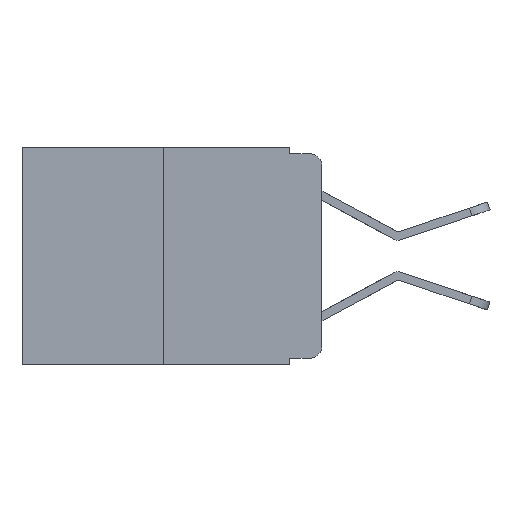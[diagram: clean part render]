
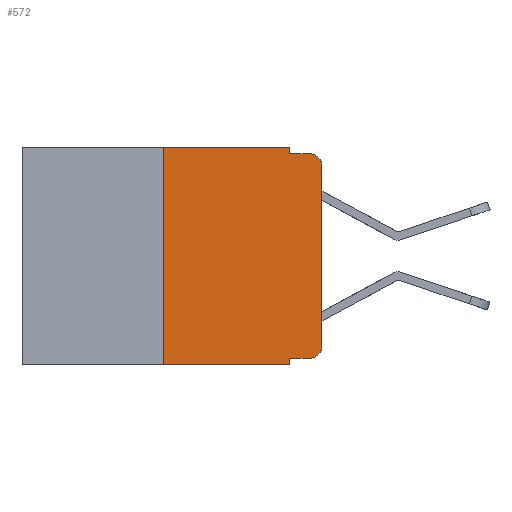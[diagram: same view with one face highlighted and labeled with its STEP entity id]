
A CAD part, left-side view. The second image highlights one B-rep face of the part: STEP entity #572.
In plain terms, the highlighted planar face has unit normal (-1, 0, 0).
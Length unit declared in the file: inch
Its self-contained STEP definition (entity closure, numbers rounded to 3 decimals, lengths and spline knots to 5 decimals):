
#12 = LINE ( 'NONE', #513, #7701 ) ;
#178 = LINE ( 'NONE', #8583, #9653 ) ;
#316 = VERTEX_POINT ( 'NONE', #3952 ) ;
#413 = DIRECTION ( 'NONE',  ( 0., 0., -1. ) ) ;
#513 = CARTESIAN_POINT ( 'NONE',  ( 0., 0.473, -0.343 ) ) ;
#572 = ADVANCED_FACE ( 'NONE', ( #7696 ), #1728, .F. ) ;
#573 = CIRCLE ( 'NONE', #2050, 0.02 ) ;
#633 = ORIENTED_EDGE ( 'NONE', *, *, #4874, .T. ) ;
#648 = ORIENTED_EDGE ( 'NONE', *, *, #5031, .T. ) ;
#751 = VECTOR ( 'NONE', #11041, 39.37008 ) ;
#838 = LINE ( 'NONE', #3670, #3539 ) ;
#1110 = ORIENTED_EDGE ( 'NONE', *, *, #4892, .F. ) ;
#1284 = DIRECTION ( 'NONE',  ( 0., 0., -1. ) ) ;
#1434 = VECTOR ( 'NONE', #4374, 39.37008 ) ;
#1572 = DIRECTION ( 'NONE',  ( 0., -1., 0. ) ) ;
#1720 = CARTESIAN_POINT ( 'NONE',  ( 0., 0.051, 0. ) ) ;
#1728 = PLANE ( 'NONE',  #8110 ) ;
#1743 = ORIENTED_EDGE ( 'NONE', *, *, #4982, .F. ) ;
#1760 = DIRECTION ( 'NONE',  ( 0., -1., 0. ) ) ;
#1807 = ORIENTED_EDGE ( 'NONE', *, *, #5016, .F. ) ;
#2050 = AXIS2_PLACEMENT_3D ( 'NONE', #3298, #6949, #1284 ) ;
#2404 = VERTEX_POINT ( 'NONE', #2656 ) ;
#2656 = CARTESIAN_POINT ( 'NONE',  ( 0., 0.25, -0.343 ) ) ;
#3298 = CARTESIAN_POINT ( 'NONE',  ( 0., 0.02, -0.03 ) ) ;
#3376 = ORIENTED_EDGE ( 'NONE', *, *, #3621, .F. ) ;
#3381 = EDGE_LOOP ( 'NONE', ( #5494, #633, #5001, #1110, #3376, #1743, #6502, #1807, #8353, #648 ) ) ;
#3450 = CARTESIAN_POINT ( 'NONE',  ( 0., 0.25, 0. ) ) ;
#3536 = CARTESIAN_POINT ( 'NONE',  ( 0., 0.051, 0. ) ) ;
#3539 = VECTOR ( 'NONE', #1760, 39.37008 ) ;
#3621 = EDGE_CURVE ( 'NONE', #316, #7828, #838, .T. ) ;
#3670 = CARTESIAN_POINT ( 'NONE',  ( 0., 0.473, 0. ) ) ;
#3745 = DIRECTION ( 'NONE',  ( -1., 0., 0. ) ) ;
#3952 = CARTESIAN_POINT ( 'NONE',  ( 0., 0.25, 0. ) ) ;
#4086 = CARTESIAN_POINT ( 'NONE',  ( 0., 0.051, -0.343 ) ) ;
#4167 = EDGE_CURVE ( 'NONE', #2404, #6299, #12, .T. ) ;
#4369 = LINE ( 'NONE', #3450, #1434 ) ;
#4374 = DIRECTION ( 'NONE',  ( 0., 0., 1. ) ) ;
#4548 = EDGE_CURVE ( 'NONE', #6968, #5547, #11079, .T. ) ;
#4633 = DIRECTION ( 'NONE',  ( 0., 0., -1. ) ) ;
#4672 = DIRECTION ( 'NONE',  ( 1., 0., 0. ) ) ;
#4874 = EDGE_CURVE ( 'NONE', #5547, #6162, #573, .T. ) ;
#4877 = EDGE_CURVE ( 'NONE', #5448, #6162, #178, .T. ) ;
#4892 = EDGE_CURVE ( 'NONE', #7828, #5448, #7560, .T. ) ;
#4982 = EDGE_CURVE ( 'NONE', #2404, #316, #4369, .T. ) ;
#5001 = ORIENTED_EDGE ( 'NONE', *, *, #4877, .F. ) ;
#5016 = EDGE_CURVE ( 'NONE', #8729, #6299, #6192, .T. ) ;
#5019 = EDGE_CURVE ( 'NONE', #8729, #9966, #8169, .T. ) ;
#5031 = EDGE_CURVE ( 'NONE', #9966, #6968, #10485, .T. ) ;
#5239 = AXIS2_PLACEMENT_3D ( 'NONE', #8963, #3745, #7965 ) ;
#5276 = CARTESIAN_POINT ( 'NONE',  ( 0., 0.02, -0.01 ) ) ;
#5448 = VERTEX_POINT ( 'NONE', #5880 ) ;
#5494 = ORIENTED_EDGE ( 'NONE', *, *, #4548, .T. ) ;
#5547 = VERTEX_POINT ( 'NONE', #10273 ) ;
#5880 = CARTESIAN_POINT ( 'NONE',  ( 0., 0.051, -0.01 ) ) ;
#5909 = VECTOR ( 'NONE', #9296, 39.37008 ) ;
#6162 = VERTEX_POINT ( 'NONE', #5276 ) ;
#6192 = LINE ( 'NONE', #3536, #5909 ) ;
#6299 = VERTEX_POINT ( 'NONE', #4086 ) ;
#6502 = ORIENTED_EDGE ( 'NONE', *, *, #4167, .T. ) ;
#6785 = DIRECTION ( 'NONE',  ( 0., -1., 0. ) ) ;
#6922 = VECTOR ( 'NONE', #10106, 39.37008 ) ;
#6949 = DIRECTION ( 'NONE',  ( -1., 0., 0. ) ) ;
#6968 = VERTEX_POINT ( 'NONE', #7885 ) ;
#7242 = CARTESIAN_POINT ( 'NONE',  ( 0., 0.051, -0.333 ) ) ;
#7469 = CARTESIAN_POINT ( 'NONE',  ( 0., 0., 0. ) ) ;
#7560 = LINE ( 'NONE', #1720, #9422 ) ;
#7696 = FACE_OUTER_BOUND ( 'NONE', #3381, .T. ) ;
#7701 = VECTOR ( 'NONE', #1572, 39.37008 ) ;
#7828 = VERTEX_POINT ( 'NONE', #10787 ) ;
#7885 = CARTESIAN_POINT ( 'NONE',  ( 0., 0., -0.313 ) ) ;
#7965 = DIRECTION ( 'NONE',  ( 0., 0., -1. ) ) ;
#8110 = AXIS2_PLACEMENT_3D ( 'NONE', #11077, #4672, #4633 ) ;
#8169 = LINE ( 'NONE', #9331, #751 ) ;
#8353 = ORIENTED_EDGE ( 'NONE', *, *, #5019, .T. ) ;
#8583 = CARTESIAN_POINT ( 'NONE',  ( 0., 0.051, -0.01 ) ) ;
#8729 = VERTEX_POINT ( 'NONE', #7242 ) ;
#8963 = CARTESIAN_POINT ( 'NONE',  ( 0., 0.02, -0.313 ) ) ;
#9296 = DIRECTION ( 'NONE',  ( 0., 0., -1. ) ) ;
#9331 = CARTESIAN_POINT ( 'NONE',  ( 0., 0.051, -0.333 ) ) ;
#9422 = VECTOR ( 'NONE', #413, 39.37008 ) ;
#9653 = VECTOR ( 'NONE', #6785, 39.37008 ) ;
#9966 = VERTEX_POINT ( 'NONE', #11499 ) ;
#10106 = DIRECTION ( 'NONE',  ( 0., 0., 1. ) ) ;
#10273 = CARTESIAN_POINT ( 'NONE',  ( 0., 0., -0.03 ) ) ;
#10485 = CIRCLE ( 'NONE', #5239, 0.02 ) ;
#10787 = CARTESIAN_POINT ( 'NONE',  ( 0., 0.051, 0. ) ) ;
#11041 = DIRECTION ( 'NONE',  ( 0., -1., 0. ) ) ;
#11077 = CARTESIAN_POINT ( 'NONE',  ( 0., 0.473, 0. ) ) ;
#11079 = LINE ( 'NONE', #7469, #6922 ) ;
#11499 = CARTESIAN_POINT ( 'NONE',  ( 0., 0.02, -0.333 ) ) ;
